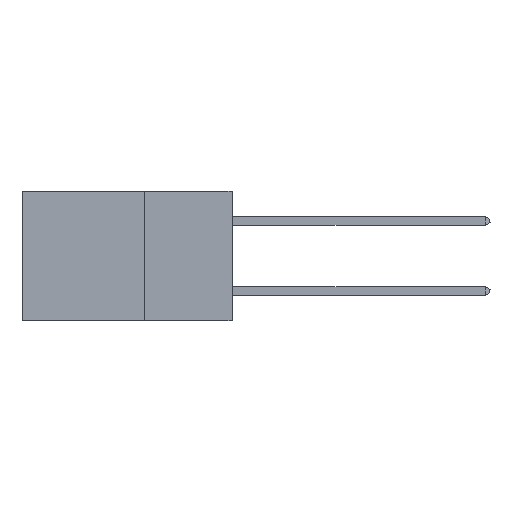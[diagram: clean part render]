
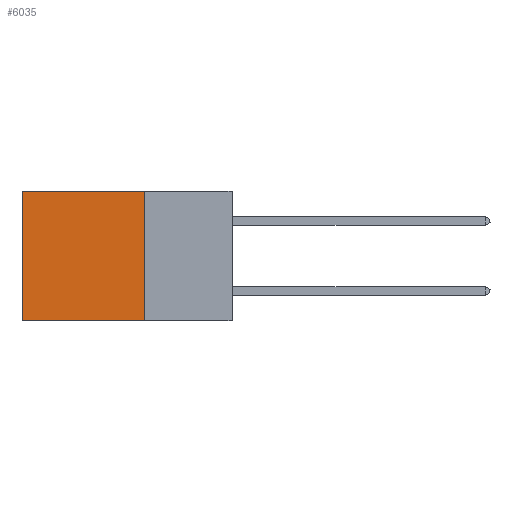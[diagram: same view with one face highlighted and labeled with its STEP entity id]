
A CAD part, left-side view. The second image highlights one B-rep face of the part: STEP entity #6035.
In plain terms, the highlighted planar face has unit normal (-1, 0, 0).
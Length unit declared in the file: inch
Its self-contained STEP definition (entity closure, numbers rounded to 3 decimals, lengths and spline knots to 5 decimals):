
#1079 = ORIENTED_EDGE ( 'NONE', *, *, #28136, .T. ) ;
#1156 = EDGE_LOOP ( 'NONE', ( #1079, #10592, #22316, #14295 ) ) ;
#3011 = CARTESIAN_POINT ( 'NONE',  ( 0.2875, 0.25, 0. ) ) ;
#4458 = CARTESIAN_POINT ( 'NONE',  ( 0.2875, 0.6, 0. ) ) ;
#5259 = VECTOR ( 'NONE', #25338, 39.37008 ) ;
#5580 = DIRECTION ( 'NONE',  ( 1., 0., 0. ) ) ;
#6035 = ADVANCED_FACE ( 'NONE', ( #15531 ), #28761, .F. ) ;
#6174 = CARTESIAN_POINT ( 'NONE',  ( 0.2875, 0.25, 0. ) ) ;
#6403 = EDGE_CURVE ( 'NONE', #7006, #28041, #6858, .T. ) ;
#6858 = LINE ( 'NONE', #6174, #26617 ) ;
#7006 = VERTEX_POINT ( 'NONE', #8266 ) ;
#8010 = CARTESIAN_POINT ( 'NONE',  ( 0.2875, 0.25, 0. ) ) ;
#8266 = CARTESIAN_POINT ( 'NONE',  ( 0.2875, 0.25, 0. ) ) ;
#8462 = AXIS2_PLACEMENT_3D ( 'NONE', #3011, #5580, #17312 ) ;
#9108 = CARTESIAN_POINT ( 'NONE',  ( 0.2875, 0.6, -0.37 ) ) ;
#10592 = ORIENTED_EDGE ( 'NONE', *, *, #12823, .F. ) ;
#11153 = CARTESIAN_POINT ( 'NONE',  ( 0.2875, 0.25, -0.37 ) ) ;
#12574 = VECTOR ( 'NONE', #14235, 39.37008 ) ;
#12823 = EDGE_CURVE ( 'NONE', #25957, #23567, #22100, .T. ) ;
#13321 = LINE ( 'NONE', #19229, #12574 ) ;
#14235 = DIRECTION ( 'NONE',  ( 0., 0., -1. ) ) ;
#14295 = ORIENTED_EDGE ( 'NONE', *, *, #6403, .T. ) ;
#15531 = FACE_OUTER_BOUND ( 'NONE', #1156, .T. ) ;
#17312 = DIRECTION ( 'NONE',  ( 0., 0., -1. ) ) ;
#17766 = VECTOR ( 'NONE', #19719, 39.37008 ) ;
#19229 = CARTESIAN_POINT ( 'NONE',  ( 0.2875, 0.6, 0. ) ) ;
#19434 = CARTESIAN_POINT ( 'NONE',  ( 0.2875, 0.25, -0.37 ) ) ;
#19719 = DIRECTION ( 'NONE',  ( 0., 0., -1. ) ) ;
#22100 = LINE ( 'NONE', #11153, #5259 ) ;
#22316 = ORIENTED_EDGE ( 'NONE', *, *, #27256, .F. ) ;
#22521 = DIRECTION ( 'NONE',  ( 0., 1., 0. ) ) ;
#23567 = VERTEX_POINT ( 'NONE', #9108 ) ;
#23954 = LINE ( 'NONE', #8010, #17766 ) ;
#25338 = DIRECTION ( 'NONE',  ( 0., 1., 0. ) ) ;
#25957 = VERTEX_POINT ( 'NONE', #19434 ) ;
#26617 = VECTOR ( 'NONE', #22521, 39.37008 ) ;
#27256 = EDGE_CURVE ( 'NONE', #7006, #25957, #23954, .T. ) ;
#28041 = VERTEX_POINT ( 'NONE', #4458 ) ;
#28136 = EDGE_CURVE ( 'NONE', #28041, #23567, #13321, .T. ) ;
#28761 = PLANE ( 'NONE',  #8462 ) ;
